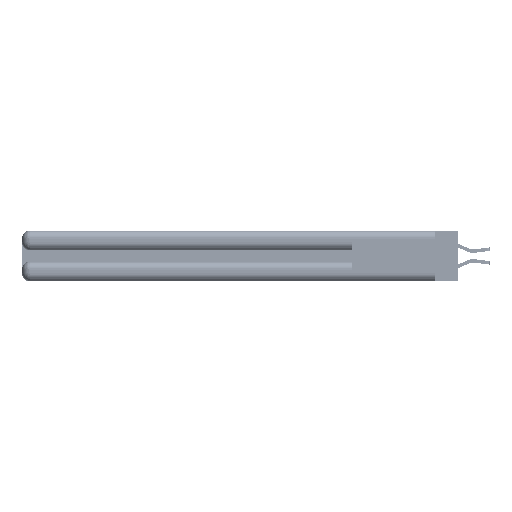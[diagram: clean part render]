
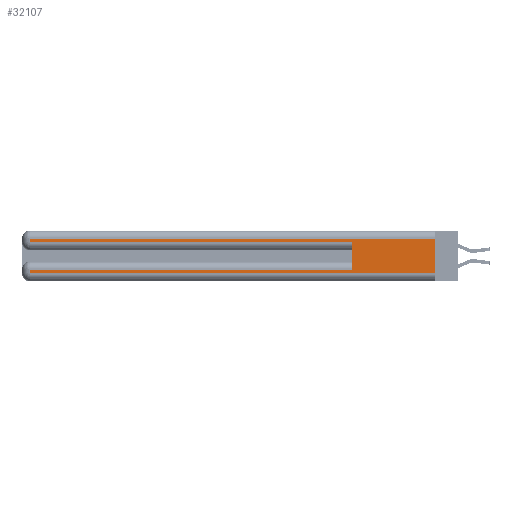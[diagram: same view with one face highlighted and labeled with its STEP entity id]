
A CAD part, left-side view. The second image highlights one B-rep face of the part: STEP entity #32107.
In plain terms, the highlighted planar face has unit normal (-1, 0, 0).
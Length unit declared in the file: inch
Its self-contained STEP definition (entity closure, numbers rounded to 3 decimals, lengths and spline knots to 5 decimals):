
#566 = CARTESIAN_POINT ( 'NONE',  ( 0., 0., 0.285 ) ) ;
#581 = EDGE_CURVE ( 'NONE', #42071, #8199, #43698, .T. ) ;
#2707 = ORIENTED_EDGE ( 'NONE', *, *, #46935, .T. ) ;
#3443 = ORIENTED_EDGE ( 'NONE', *, *, #36231, .T. ) ;
#4743 = ORIENTED_EDGE ( 'NONE', *, *, #25462, .T. ) ;
#5735 = CARTESIAN_POINT ( 'NONE',  ( 0., 0., 0.31 ) ) ;
#6240 = EDGE_LOOP ( 'NONE', ( #11648, #21295, #38256, #46769, #39676, #4743, #3443, #2707 ) ) ;
#8199 = VERTEX_POINT ( 'NONE', #29423 ) ;
#8531 = VECTOR ( 'NONE', #41088, 39.37008 ) ;
#8723 = CARTESIAN_POINT ( 'NONE',  ( 0., 0., 0.37 ) ) ;
#9620 = LINE ( 'NONE', #34247, #51816 ) ;
#10828 = CARTESIAN_POINT ( 'NONE',  ( 0., 0., 0.06 ) ) ;
#11581 = CARTESIAN_POINT ( 'NONE',  ( 0., 0., 0.31 ) ) ;
#11648 = ORIENTED_EDGE ( 'NONE', *, *, #37997, .F. ) ;
#11942 = VERTEX_POINT ( 'NONE', #43827 ) ;
#12301 = CARTESIAN_POINT ( 'NONE',  ( 0., 0., 0.37 ) ) ;
#12851 = DIRECTION ( 'NONE',  ( 0., 0., -1. ) ) ;
#13594 = VECTOR ( 'NONE', #24077, 39.37008 ) ;
#13863 = DIRECTION ( 'NONE',  ( 0., 1., 0. ) ) ;
#14047 = EDGE_CURVE ( 'NONE', #18411, #36790, #49398, .T. ) ;
#16012 = VERTEX_POINT ( 'NONE', #10828 ) ;
#16419 = DIRECTION ( 'NONE',  ( 0., 0., -1. ) ) ;
#16499 = LINE ( 'NONE', #11581, #36954 ) ;
#17247 = LINE ( 'NONE', #8723, #37702 ) ;
#17567 = EDGE_CURVE ( 'NONE', #28902, #42071, #16499, .T. ) ;
#18411 = VERTEX_POINT ( 'NONE', #47493 ) ;
#21295 = ORIENTED_EDGE ( 'NONE', *, *, #17567, .T. ) ;
#22458 = DIRECTION ( 'NONE',  ( 0., 0., -1. ) ) ;
#24077 = DIRECTION ( 'NONE',  ( 0., -1., 0. ) ) ;
#25028 = DIRECTION ( 'NONE',  ( 0., -1., 0. ) ) ;
#25462 = EDGE_CURVE ( 'NONE', #18411, #11942, #9620, .T. ) ;
#28205 = CARTESIAN_POINT ( 'NONE',  ( 0., 0., 0.06 ) ) ;
#28463 = CARTESIAN_POINT ( 'NONE',  ( 0., 0.6, 0.145 ) ) ;
#28636 = DIRECTION ( 'NONE',  ( 0., 0., 1. ) ) ;
#28902 = VERTEX_POINT ( 'NONE', #5735 ) ;
#29423 = CARTESIAN_POINT ( 'NONE',  ( 0., 2.94, 0.285 ) ) ;
#29665 = AXIS2_PLACEMENT_3D ( 'NONE', #12301, #40889, #16419 ) ;
#31415 = VECTOR ( 'NONE', #25028, 39.37008 ) ;
#31882 = CARTESIAN_POINT ( 'NONE',  ( 0., 2.94, 0.06 ) ) ;
#32107 = ADVANCED_FACE ( 'NONE', ( #47468 ), #36798, .F. ) ;
#34223 = CARTESIAN_POINT ( 'NONE',  ( 0., 0.6, 0.285 ) ) ;
#34247 = CARTESIAN_POINT ( 'NONE',  ( 0., 0., 0.085 ) ) ;
#35711 = CARTESIAN_POINT ( 'NONE',  ( 0., 2.94, 0.31 ) ) ;
#36058 = DIRECTION ( 'NONE',  ( 0., 1., 0. ) ) ;
#36231 = EDGE_CURVE ( 'NONE', #11942, #40968, #48169, .T. ) ;
#36790 = VERTEX_POINT ( 'NONE', #34223 ) ;
#36798 = PLANE ( 'NONE',  #29665 ) ;
#36954 = VECTOR ( 'NONE', #36058, 39.37008 ) ;
#37243 = EDGE_CURVE ( 'NONE', #8199, #36790, #40988, .T. ) ;
#37301 = VECTOR ( 'NONE', #22458, 39.37008 ) ;
#37702 = VECTOR ( 'NONE', #12851, 39.37008 ) ;
#37997 = EDGE_CURVE ( 'NONE', #28902, #16012, #17247, .T. ) ;
#38256 = ORIENTED_EDGE ( 'NONE', *, *, #581, .T. ) ;
#38512 = VECTOR ( 'NONE', #28636, 39.37008 ) ;
#38740 = CARTESIAN_POINT ( 'NONE',  ( 0., 2.94, 0.37 ) ) ;
#39676 = ORIENTED_EDGE ( 'NONE', *, *, #14047, .F. ) ;
#40889 = DIRECTION ( 'NONE',  ( 1., 0., 0. ) ) ;
#40968 = VERTEX_POINT ( 'NONE', #31882 ) ;
#40988 = LINE ( 'NONE', #566, #31415 ) ;
#41088 = DIRECTION ( 'NONE',  ( 0., 0., -1. ) ) ;
#42071 = VERTEX_POINT ( 'NONE', #35711 ) ;
#43698 = LINE ( 'NONE', #50199, #8531 ) ;
#43827 = CARTESIAN_POINT ( 'NONE',  ( 0., 2.94, 0.085 ) ) ;
#46183 = LINE ( 'NONE', #28205, #13594 ) ;
#46769 = ORIENTED_EDGE ( 'NONE', *, *, #37243, .T. ) ;
#46935 = EDGE_CURVE ( 'NONE', #40968, #16012, #46183, .T. ) ;
#47468 = FACE_OUTER_BOUND ( 'NONE', #6240, .T. ) ;
#47493 = CARTESIAN_POINT ( 'NONE',  ( 0., 0.6, 0.085 ) ) ;
#48169 = LINE ( 'NONE', #38740, #37301 ) ;
#49398 = LINE ( 'NONE', #28463, #38512 ) ;
#50199 = CARTESIAN_POINT ( 'NONE',  ( 0., 2.94, 0.37 ) ) ;
#51816 = VECTOR ( 'NONE', #13863, 39.37008 ) ;
